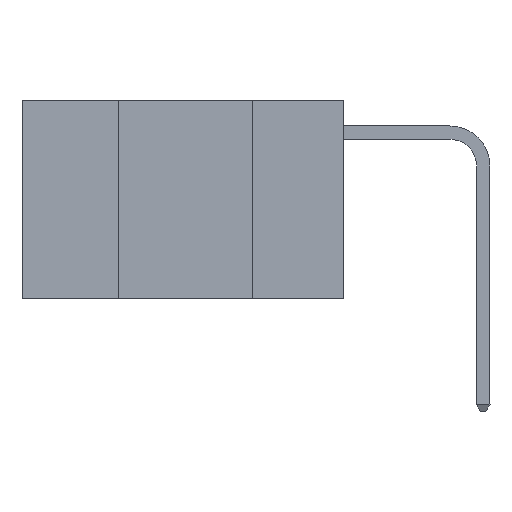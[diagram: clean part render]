
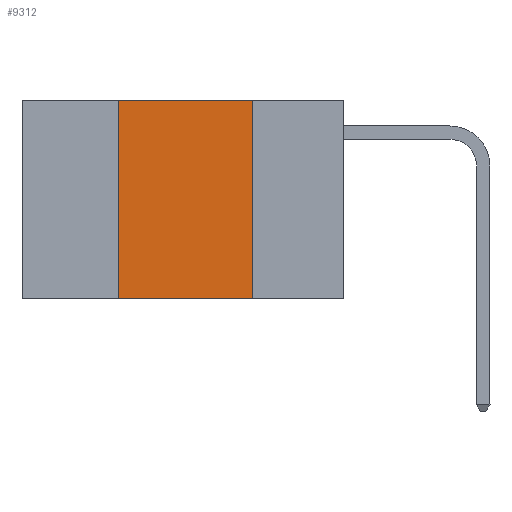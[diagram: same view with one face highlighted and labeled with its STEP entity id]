
A CAD part, left-side view. The second image highlights one B-rep face of the part: STEP entity #9312.
In plain terms, the highlighted planar face has unit normal (-1, 0, 0).
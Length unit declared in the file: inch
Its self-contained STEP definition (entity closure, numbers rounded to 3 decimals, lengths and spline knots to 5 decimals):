
#62 = VECTOR ( 'NONE', #4456, 39.37008 ) ;
#99 = VECTOR ( 'NONE', #2922, 39.37008 ) ;
#122 = AXIS2_PLACEMENT_3D ( 'NONE', #11890, #3966, #11937 ) ;
#220 = EDGE_CURVE ( 'NONE', #12398, #8493, #7224, .T. ) ;
#570 = ORIENTED_EDGE ( 'NONE', *, *, #220, .T. ) ;
#1001 = EDGE_CURVE ( 'NONE', #8779, #8493, #11626, .T. ) ;
#1490 = EDGE_LOOP ( 'NONE', ( #4229, #10657, #9065, #570 ) ) ;
#2382 = CARTESIAN_POINT ( 'NONE',  ( 0., 0.42, 0. ) ) ;
#2590 = EDGE_CURVE ( 'NONE', #12398, #3384, #3192, .T. ) ;
#2891 = LINE ( 'NONE', #12590, #5636 ) ;
#2922 = DIRECTION ( 'NONE',  ( 0., 0., -1. ) ) ;
#3113 = FACE_OUTER_BOUND ( 'NONE', #1490, .T. ) ;
#3192 = LINE ( 'NONE', #5643, #62 ) ;
#3384 = VERTEX_POINT ( 'NONE', #2382 ) ;
#3544 = CARTESIAN_POINT ( 'NONE',  ( 0., 0.17, -0.37 ) ) ;
#3966 = DIRECTION ( 'NONE',  ( 1., 0., 0. ) ) ;
#4229 = ORIENTED_EDGE ( 'NONE', *, *, #1001, .F. ) ;
#4456 = DIRECTION ( 'NONE',  ( 0., 0., 1. ) ) ;
#4650 = DIRECTION ( 'NONE',  ( 0., -1., 0. ) ) ;
#4753 = CARTESIAN_POINT ( 'NONE',  ( 0., 0.6, -0.37 ) ) ;
#5270 = DIRECTION ( 'NONE',  ( 0., -1., 0. ) ) ;
#5636 = VECTOR ( 'NONE', #4650, 39.37008 ) ;
#5643 = CARTESIAN_POINT ( 'NONE',  ( 0., 0.42, 0. ) ) ;
#5910 = CARTESIAN_POINT ( 'NONE',  ( 0., 0.42, -0.37 ) ) ;
#6447 = EDGE_CURVE ( 'NONE', #3384, #8779, #2891, .T. ) ;
#7224 = LINE ( 'NONE', #4753, #9877 ) ;
#7506 = CARTESIAN_POINT ( 'NONE',  ( 0., 0.17, 0. ) ) ;
#8493 = VERTEX_POINT ( 'NONE', #3544 ) ;
#8779 = VERTEX_POINT ( 'NONE', #7506 ) ;
#9065 = ORIENTED_EDGE ( 'NONE', *, *, #2590, .F. ) ;
#9312 = ADVANCED_FACE ( 'NONE', ( #3113 ), #9668, .F. ) ;
#9668 = PLANE ( 'NONE',  #122 ) ;
#9877 = VECTOR ( 'NONE', #5270, 39.37008 ) ;
#10657 = ORIENTED_EDGE ( 'NONE', *, *, #6447, .F. ) ;
#10926 = CARTESIAN_POINT ( 'NONE',  ( 0., 0.17, 0. ) ) ;
#11626 = LINE ( 'NONE', #10926, #99 ) ;
#11890 = CARTESIAN_POINT ( 'NONE',  ( 0., 0.6, 0. ) ) ;
#11937 = DIRECTION ( 'NONE',  ( 0., 0., -1. ) ) ;
#12398 = VERTEX_POINT ( 'NONE', #5910 ) ;
#12590 = CARTESIAN_POINT ( 'NONE',  ( 0., 0.6, 0. ) ) ;
